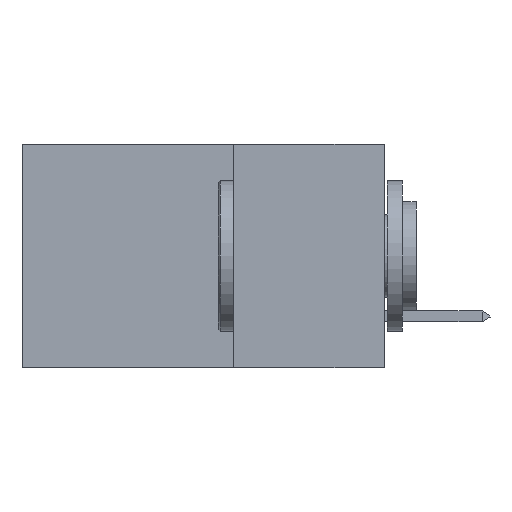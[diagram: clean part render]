
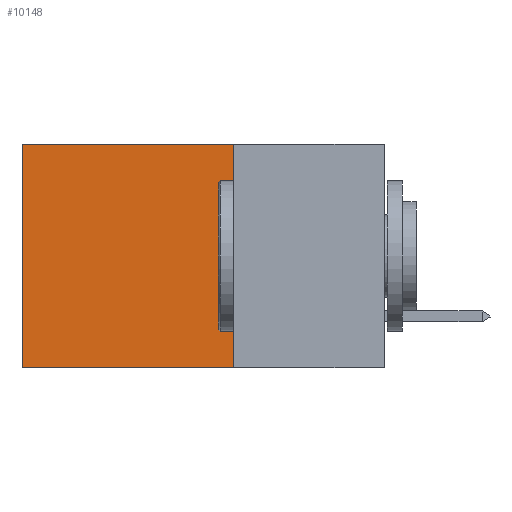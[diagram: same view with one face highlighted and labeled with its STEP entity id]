
A CAD part, left-side view. The second image highlights one B-rep face of the part: STEP entity #10148.
In plain terms, the highlighted planar face has unit normal (-1, 0, 0).
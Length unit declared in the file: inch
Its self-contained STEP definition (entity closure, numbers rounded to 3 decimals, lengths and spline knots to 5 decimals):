
#107 = LINE ( 'NONE', #16540, #1328 ) ;
#761 = DIRECTION ( 'NONE',  ( 0., 1., 0. ) ) ;
#1328 = VECTOR ( 'NONE', #8803, 39.37008 ) ;
#1752 = EDGE_CURVE ( 'NONE', #7560, #20586, #107, .T. ) ;
#1956 = CARTESIAN_POINT ( 'NONE',  ( 0.2875, 0.25, -0.37 ) ) ;
#2562 = CARTESIAN_POINT ( 'NONE',  ( 0.2875, 0.6, -0.37 ) ) ;
#2933 = EDGE_CURVE ( 'NONE', #7560, #9369, #8489, .T. ) ;
#3537 = VECTOR ( 'NONE', #7329, 39.37008 ) ;
#3707 = DIRECTION ( 'NONE',  ( 0., 0., -1. ) ) ;
#4228 = VERTEX_POINT ( 'NONE', #2562 ) ;
#5147 = EDGE_CURVE ( 'NONE', #9369, #4228, #17439, .T. ) ;
#5343 = CARTESIAN_POINT ( 'NONE',  ( 0.2875, 0.25, -0.37 ) ) ;
#6490 = ORIENTED_EDGE ( 'NONE', *, *, #5147, .T. ) ;
#6577 = VECTOR ( 'NONE', #3707, 39.37008 ) ;
#6893 = DIRECTION ( 'NONE',  ( 1., 0., 0. ) ) ;
#7329 = DIRECTION ( 'NONE',  ( 0., 1., 0. ) ) ;
#7560 = VERTEX_POINT ( 'NONE', #8193 ) ;
#8193 = CARTESIAN_POINT ( 'NONE',  ( 0.2875, 0.25, 0. ) ) ;
#8489 = LINE ( 'NONE', #21787, #19071 ) ;
#8803 = DIRECTION ( 'NONE',  ( 0., 0., -1. ) ) ;
#9201 = ORIENTED_EDGE ( 'NONE', *, *, #2933, .T. ) ;
#9369 = VERTEX_POINT ( 'NONE', #9586 ) ;
#9586 = CARTESIAN_POINT ( 'NONE',  ( 0.2875, 0.6, 0. ) ) ;
#10148 = ADVANCED_FACE ( 'NONE', ( #11027 ), #14820, .F. ) ;
#11027 = FACE_OUTER_BOUND ( 'NONE', #13584, .T. ) ;
#12623 = CARTESIAN_POINT ( 'NONE',  ( 0.2875, 0.25, 0. ) ) ;
#13584 = EDGE_LOOP ( 'NONE', ( #6490, #17310, #16692, #9201 ) ) ;
#14324 = EDGE_CURVE ( 'NONE', #20586, #4228, #15600, .T. ) ;
#14820 = PLANE ( 'NONE',  #22661 ) ;
#15600 = LINE ( 'NONE', #5343, #3537 ) ;
#16540 = CARTESIAN_POINT ( 'NONE',  ( 0.2875, 0.25, 0. ) ) ;
#16692 = ORIENTED_EDGE ( 'NONE', *, *, #1752, .F. ) ;
#17310 = ORIENTED_EDGE ( 'NONE', *, *, #14324, .F. ) ;
#17439 = LINE ( 'NONE', #19246, #6577 ) ;
#19071 = VECTOR ( 'NONE', #761, 39.37008 ) ;
#19246 = CARTESIAN_POINT ( 'NONE',  ( 0.2875, 0.6, 0. ) ) ;
#20586 = VERTEX_POINT ( 'NONE', #1956 ) ;
#21787 = CARTESIAN_POINT ( 'NONE',  ( 0.2875, 0.25, 0. ) ) ;
#22334 = DIRECTION ( 'NONE',  ( 0., 0., -1. ) ) ;
#22661 = AXIS2_PLACEMENT_3D ( 'NONE', #12623, #6893, #22334 ) ;
